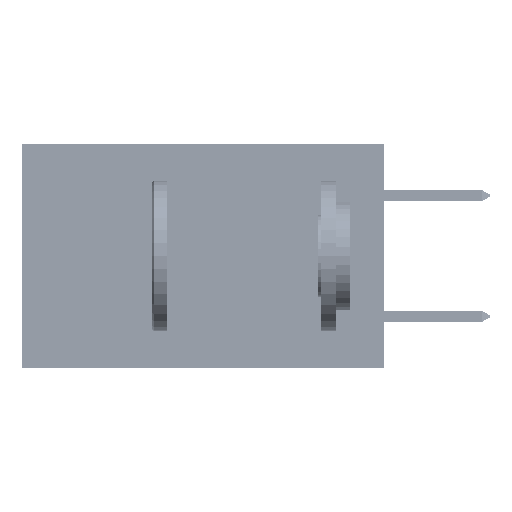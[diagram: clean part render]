
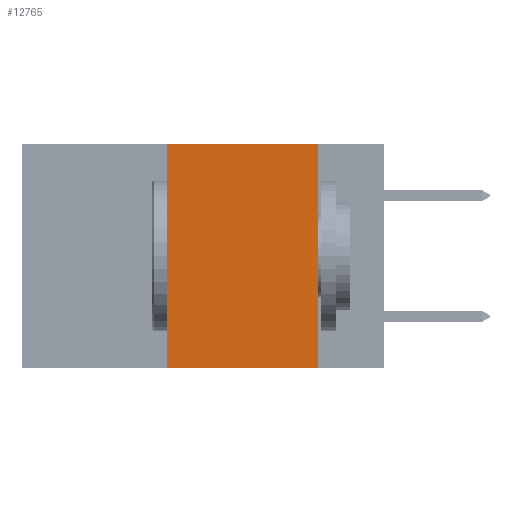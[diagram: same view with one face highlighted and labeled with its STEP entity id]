
A CAD part, left-side view. The second image highlights one B-rep face of the part: STEP entity #12765.
In plain terms, the highlighted planar face has unit normal (-1, 0, 0).
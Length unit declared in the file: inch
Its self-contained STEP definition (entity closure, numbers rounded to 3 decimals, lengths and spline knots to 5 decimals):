
#71 = CARTESIAN_POINT ( 'NONE',  ( 0., 0.6, 0. ) ) ;
#240 = DIRECTION ( 'NONE',  ( 0., 0., -1. ) ) ;
#2921 = VERTEX_POINT ( 'NONE', #39477 ) ;
#2951 = AXIS2_PLACEMENT_3D ( 'NONE', #71, #22780, #240 ) ;
#5107 = EDGE_CURVE ( 'NONE', #2921, #29050, #41207, .T. ) ;
#8229 = EDGE_LOOP ( 'NONE', ( #18977, #12522, #37504, #19787 ) ) ;
#8265 = LINE ( 'NONE', #11887, #36752 ) ;
#8693 = EDGE_CURVE ( 'NONE', #29050, #18479, #41450, .T. ) ;
#11887 = CARTESIAN_POINT ( 'NONE',  ( 0., 0.6, -0.37 ) ) ;
#12522 = ORIENTED_EDGE ( 'NONE', *, *, #8693, .F. ) ;
#12765 = ADVANCED_FACE ( 'NONE', ( #34074 ), #41154, .F. ) ;
#15181 = VECTOR ( 'NONE', #44315, 39.37008 ) ;
#15623 = DIRECTION ( 'NONE',  ( 0., 0., -1. ) ) ;
#17271 = VECTOR ( 'NONE', #15623, 39.37008 ) ;
#17852 = CARTESIAN_POINT ( 'NONE',  ( 0., 0.6, 0. ) ) ;
#18479 = VERTEX_POINT ( 'NONE', #43933 ) ;
#18977 = ORIENTED_EDGE ( 'NONE', *, *, #47374, .F. ) ;
#19787 = ORIENTED_EDGE ( 'NONE', *, *, #23595, .T. ) ;
#21570 = DIRECTION ( 'NONE',  ( 0., -1., 0. ) ) ;
#21827 = VECTOR ( 'NONE', #21570, 39.37008 ) ;
#22168 = VERTEX_POINT ( 'NONE', #40188 ) ;
#22780 = DIRECTION ( 'NONE',  ( 1., 0., 0. ) ) ;
#23595 = EDGE_CURVE ( 'NONE', #2921, #22168, #8265, .T. ) ;
#27885 = CARTESIAN_POINT ( 'NONE',  ( 0., 0.36, 0. ) ) ;
#28292 = LINE ( 'NONE', #34092, #17271 ) ;
#29050 = VERTEX_POINT ( 'NONE', #27885 ) ;
#34074 = FACE_OUTER_BOUND ( 'NONE', #8229, .T. ) ;
#34092 = CARTESIAN_POINT ( 'NONE',  ( 0., 0.11, 0. ) ) ;
#36752 = VECTOR ( 'NONE', #37829, 39.37008 ) ;
#37504 = ORIENTED_EDGE ( 'NONE', *, *, #5107, .F. ) ;
#37829 = DIRECTION ( 'NONE',  ( 0., -1., 0. ) ) ;
#39477 = CARTESIAN_POINT ( 'NONE',  ( 0., 0.36, -0.37 ) ) ;
#40188 = CARTESIAN_POINT ( 'NONE',  ( 0., 0.11, -0.37 ) ) ;
#40614 = CARTESIAN_POINT ( 'NONE',  ( 0., 0.36, 0. ) ) ;
#41154 = PLANE ( 'NONE',  #2951 ) ;
#41207 = LINE ( 'NONE', #40614, #15181 ) ;
#41450 = LINE ( 'NONE', #17852, #21827 ) ;
#43933 = CARTESIAN_POINT ( 'NONE',  ( 0., 0.11, 0. ) ) ;
#44315 = DIRECTION ( 'NONE',  ( 0., 0., 1. ) ) ;
#47374 = EDGE_CURVE ( 'NONE', #18479, #22168, #28292, .T. ) ;
